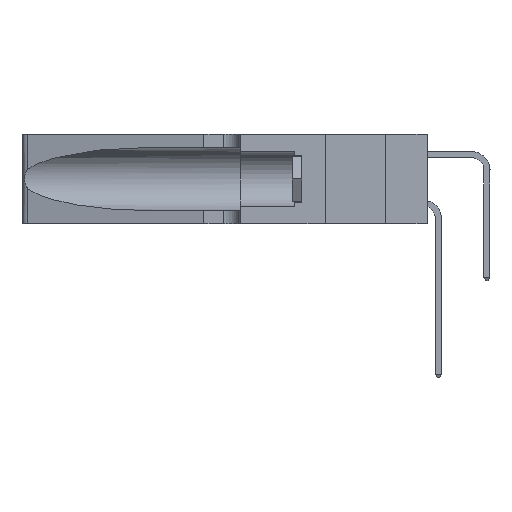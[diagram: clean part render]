
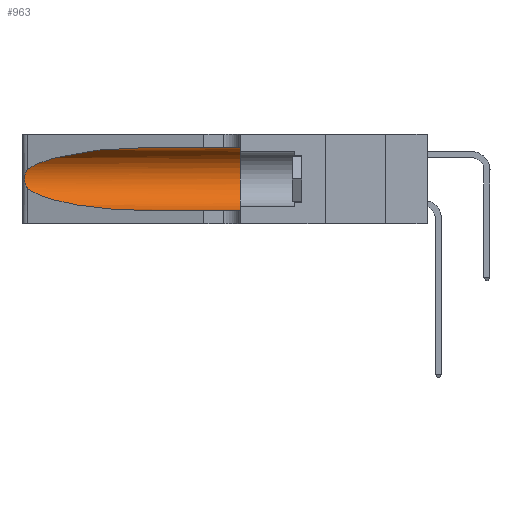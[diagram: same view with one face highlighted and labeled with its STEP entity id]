
A CAD part, left-side view. The second image highlights one B-rep face of the part: STEP entity #963.
In plain terms, the highlighted cylindrical face has radius 3.308 mm (diameter 6.617 mm), a partial arc.
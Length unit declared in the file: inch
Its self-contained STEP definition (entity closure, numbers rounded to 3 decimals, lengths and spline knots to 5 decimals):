
#303 = VERTEX_POINT ( 'NONE', #31771 ) ;
#963 = ADVANCED_FACE ( 'NONE', ( #37491 ), #19097, .F. ) ;
#1042 = VERTEX_POINT ( 'NONE', #26365 ) ;
#2464 = CARTESIAN_POINT ( 'NONE',  ( 0.25787, 1.23484, 0.2124 ) ) ;
#3819 = CARTESIAN_POINT ( 'NONE',  ( 0.2373, 1.15595, 0.28018 ) ) ;
#4390 = CARTESIAN_POINT ( 'NONE',  ( 0.1305, 1.61858, 0.185 ) ) ;
#4588 = CARTESIAN_POINT ( 'NONE',  ( 0.1305, 0.72297, 0.05475 ) ) ;
#5604 = CARTESIAN_POINT ( 'NONE',  ( 0.26018, 1.23835, 0.19895 ) ) ;
#7494 = DIRECTION ( 'NONE',  ( 0., 0., -1. ) ) ;
#7797 = VECTOR ( 'NONE', #14601, 39.37008 ) ;
#7963 = B_SPLINE_CURVE_WITH_KNOTS ( 'NONE', 3,
 ( #14862, #33390, #21089, #2464, #24220, #5604, #27299, #8725, #30378, #11867, #33530, #14998, #36638, #18125 ),
 .UNSPECIFIED., .F., .F.,
 ( 4, 2, 2, 2, 2, 2, 4 ),
 ( 0., 0.00027, 0.00053, 0.00107, 0.0016, 0.00187, 0.00214 ),
 .UNSPECIFIED. ) ;
#8549 = VERTEX_POINT ( 'NONE', #22562 ) ;
#8725 = CARTESIAN_POINT ( 'NONE',  ( 0.26075, 1.23896, 0.178 ) ) ;
#11352 = CARTESIAN_POINT ( 'NONE',  ( 0.1305, 0.35, 0.05475 ) ) ;
#11867 = CARTESIAN_POINT ( 'NONE',  ( 0.25856, 1.23593, 0.16098 ) ) ;
#11970 = DIRECTION ( 'NONE',  ( 0., 1., 0. ) ) ;
#13774 = DIRECTION ( 'NONE',  ( 0., -1., 0. ) ) ;
#13825 = CARTESIAN_POINT ( 'NONE',  ( 0.2373, 1.15595, 0.08982 ) ) ;
#14181 = EDGE_LOOP ( 'NONE', ( #21263, #35031, #25105, #34748, #19568, #30209 ) ) ;
#14601 = DIRECTION ( 'NONE',  ( 0., -1., 0. ) ) ;
#14862 = CARTESIAN_POINT ( 'NONE',  ( 0.25487, 1.22718, 0.22369 ) ) ;
#14998 = CARTESIAN_POINT ( 'NONE',  ( 0.25639, 1.23186, 0.15144 ) ) ;
#15010 = EDGE_CURVE ( 'NONE', #8549, #24306, #7963, .T. ) ;
#15239 = AXIS2_PLACEMENT_3D ( 'NONE', #4390, #13774, #7494 ) ;
#15831 =( BOUNDED_CURVE ( )  B_SPLINE_CURVE ( 3, ( #20044, #13825, #23175, #4588 ),
 .UNSPECIFIED., .F., .T. ) 
 B_SPLINE_CURVE_WITH_KNOTS ( ( 4, 4 ),
 ( 3.44316, 4.71239 ),
 .UNSPECIFIED. ) 
 CURVE ( )  GEOMETRIC_REPRESENTATION_ITEM ( )  RATIONAL_B_SPLINE_CURVE ( ( 1., 0.87, 0.87, 1. ) ) 
 REPRESENTATION_ITEM ( '' )  );
#16220 = CARTESIAN_POINT ( 'NONE',  ( 0.1305, 0.72297, 0.31525 ) ) ;
#17210 = CARTESIAN_POINT ( 'NONE',  ( 0.1305, 1.61858, 0.31525 ) ) ;
#18125 = CARTESIAN_POINT ( 'NONE',  ( 0.25487, 1.22718, 0.14631 ) ) ;
#19097 = CYLINDRICAL_SURFACE ( 'NONE', #15239, 0.13025 ) ;
#19568 = ORIENTED_EDGE ( 'NONE', *, *, #38002, .F. ) ;
#20044 = CARTESIAN_POINT ( 'NONE',  ( 0.25487, 1.22718, 0.14631 ) ) ;
#20891 = AXIS2_PLACEMENT_3D ( 'NONE', #30479, #11970, #33625 ) ;
#21089 = CARTESIAN_POINT ( 'NONE',  ( 0.25639, 1.23184, 0.21858 ) ) ;
#21195 = LINE ( 'NONE', #17210, #37635 ) ;
#21263 = ORIENTED_EDGE ( 'NONE', *, *, #31245, .T. ) ;
#21532 =( BOUNDED_CURVE ( )  B_SPLINE_CURVE ( 3, ( #16220, #34729, #3819, #25564 ),
 .UNSPECIFIED., .F., .F. ) 
 B_SPLINE_CURVE_WITH_KNOTS ( ( 4, 4 ),
 ( 1.5708, 2.84003 ),
 .UNSPECIFIED. ) 
 CURVE ( )  GEOMETRIC_REPRESENTATION_ITEM ( )  RATIONAL_B_SPLINE_CURVE ( ( 1., 0.87, 0.87, 1. ) ) 
 REPRESENTATION_ITEM ( '' )  );
#22562 = CARTESIAN_POINT ( 'NONE',  ( 0.25487, 1.22718, 0.22369 ) ) ;
#23175 = CARTESIAN_POINT ( 'NONE',  ( 0.18966, 0.96281, 0.05475 ) ) ;
#23369 = LINE ( 'NONE', #27053, #7797 ) ;
#23970 = VERTEX_POINT ( 'NONE', #11352 ) ;
#24220 = CARTESIAN_POINT ( 'NONE',  ( 0.25854, 1.2359, 0.20912 ) ) ;
#24306 = VERTEX_POINT ( 'NONE', #37718 ) ;
#25105 = ORIENTED_EDGE ( 'NONE', *, *, #28506, .T. ) ;
#25564 = CARTESIAN_POINT ( 'NONE',  ( 0.25487, 1.22718, 0.22369 ) ) ;
#26360 = CIRCLE ( 'NONE', #20891, 0.13025 ) ;
#26365 = CARTESIAN_POINT ( 'NONE',  ( 0.1305, 0.72297, 0.31525 ) ) ;
#27053 = CARTESIAN_POINT ( 'NONE',  ( 0.1305, 1.61858, 0.05475 ) ) ;
#27299 = CARTESIAN_POINT ( 'NONE',  ( 0.26075, 1.23896, 0.19203 ) ) ;
#28506 = EDGE_CURVE ( 'NONE', #24306, #34920, #15831, .T. ) ;
#29732 = CARTESIAN_POINT ( 'NONE',  ( 0.1305, 0.72297, 0.05475 ) ) ;
#30209 = ORIENTED_EDGE ( 'NONE', *, *, #34304, .F. ) ;
#30378 = CARTESIAN_POINT ( 'NONE',  ( 0.26017, 1.23833, 0.17102 ) ) ;
#30479 = CARTESIAN_POINT ( 'NONE',  ( 0.1305, 0.35, 0.185 ) ) ;
#30864 = EDGE_CURVE ( 'NONE', #34920, #23970, #23369, .T. ) ;
#31245 = EDGE_CURVE ( 'NONE', #1042, #8549, #21532, .T. ) ;
#31771 = CARTESIAN_POINT ( 'NONE',  ( 0.1305, 0.35, 0.31525 ) ) ;
#33390 = CARTESIAN_POINT ( 'NONE',  ( 0.25555, 1.22994, 0.2215 ) ) ;
#33530 = CARTESIAN_POINT ( 'NONE',  ( 0.25789, 1.23486, 0.15765 ) ) ;
#33625 = DIRECTION ( 'NONE',  ( 0., 0., 1. ) ) ;
#34304 = EDGE_CURVE ( 'NONE', #1042, #303, #21195, .T. ) ;
#34729 = CARTESIAN_POINT ( 'NONE',  ( 0.18966, 0.96281, 0.31525 ) ) ;
#34748 = ORIENTED_EDGE ( 'NONE', *, *, #30864, .T. ) ;
#34920 = VERTEX_POINT ( 'NONE', #29732 ) ;
#35031 = ORIENTED_EDGE ( 'NONE', *, *, #15010, .T. ) ;
#36638 = CARTESIAN_POINT ( 'NONE',  ( 0.25555, 1.22993, 0.14849 ) ) ;
#37491 = FACE_OUTER_BOUND ( 'NONE', #14181, .T. ) ;
#37635 = VECTOR ( 'NONE', #38826, 39.37008 ) ;
#37718 = CARTESIAN_POINT ( 'NONE',  ( 0.25487, 1.22718, 0.14631 ) ) ;
#38002 = EDGE_CURVE ( 'NONE', #303, #23970, #26360, .T. ) ;
#38826 = DIRECTION ( 'NONE',  ( 0., -1., 0. ) ) ;
